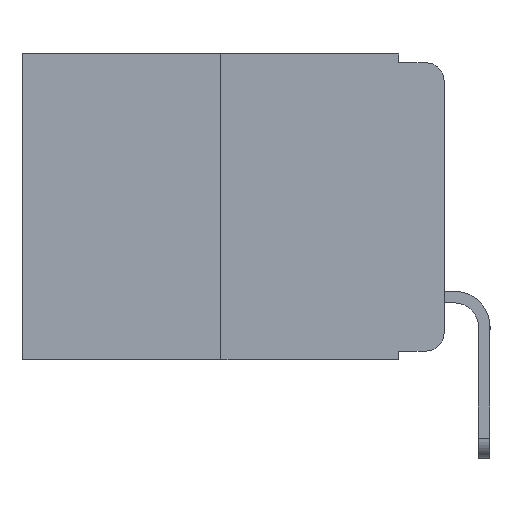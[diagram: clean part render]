
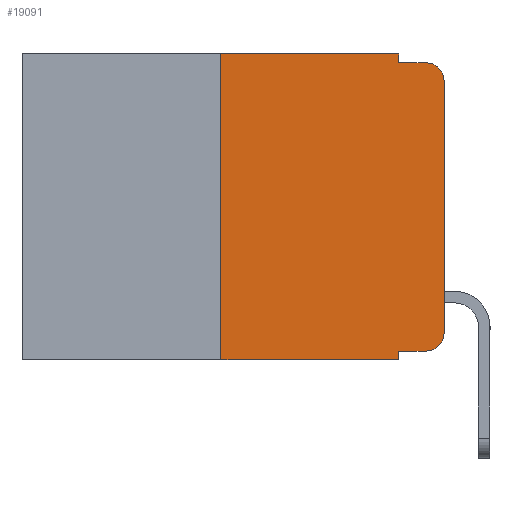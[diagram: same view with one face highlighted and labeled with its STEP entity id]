
A CAD part, left-side view. The second image highlights one B-rep face of the part: STEP entity #19091.
In plain terms, the highlighted planar face has unit normal (-1, 0, 0).
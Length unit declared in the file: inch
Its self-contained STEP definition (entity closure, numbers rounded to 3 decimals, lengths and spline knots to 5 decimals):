
#580 = LINE ( 'NONE', #835, #15946 ) ;
#835 = CARTESIAN_POINT ( 'NONE',  ( 0., 0.051, -0.01 ) ) ;
#1684 = VERTEX_POINT ( 'NONE', #20459 ) ;
#1889 = PLANE ( 'NONE',  #7330 ) ;
#2268 = EDGE_CURVE ( 'NONE', #1684, #6836, #22344, .T. ) ;
#2276 = DIRECTION ( 'NONE',  ( -1., 0., 0. ) ) ;
#2827 = VERTEX_POINT ( 'NONE', #14921 ) ;
#3112 = CARTESIAN_POINT ( 'NONE',  ( 0., 0., 0. ) ) ;
#3487 = CARTESIAN_POINT ( 'NONE',  ( 0., 0.25, -0.343 ) ) ;
#4690 = VECTOR ( 'NONE', #24886, 39.37008 ) ;
#4863 = CARTESIAN_POINT ( 'NONE',  ( 0., 0.02, -0.01 ) ) ;
#5251 = VECTOR ( 'NONE', #22073, 39.37008 ) ;
#5925 = LINE ( 'NONE', #6495, #5251 ) ;
#6188 = VECTOR ( 'NONE', #21374, 39.37008 ) ;
#6495 = CARTESIAN_POINT ( 'NONE',  ( 0., 0.473, -0.343 ) ) ;
#6691 = AXIS2_PLACEMENT_3D ( 'NONE', #9468, #22991, #11340 ) ;
#6836 = VERTEX_POINT ( 'NONE', #24330 ) ;
#7007 = VECTOR ( 'NONE', #13917, 39.37008 ) ;
#7330 = AXIS2_PLACEMENT_3D ( 'NONE', #16292, #10390, #23853 ) ;
#7694 = CARTESIAN_POINT ( 'NONE',  ( 0., 0.051, 0. ) ) ;
#8167 = EDGE_CURVE ( 'NONE', #10676, #2827, #22219, .T. ) ;
#8172 = EDGE_CURVE ( 'NONE', #2827, #24056, #17163, .T. ) ;
#8215 = EDGE_CURVE ( 'NONE', #19932, #24056, #580, .T. ) ;
#8297 = EDGE_CURVE ( 'NONE', #6836, #19932, #25761, .T. ) ;
#8474 = EDGE_CURVE ( 'NONE', #20167, #1684, #18103, .T. ) ;
#8585 = EDGE_CURVE ( 'NONE', #19271, #10582, #20757, .T. ) ;
#8639 = VERTEX_POINT ( 'NONE', #18443 ) ;
#8981 = CARTESIAN_POINT ( 'NONE',  ( 0., 0.051, -0.333 ) ) ;
#9074 = CIRCLE ( 'NONE', #20930, 0.02 ) ;
#9227 = EDGE_CURVE ( 'NONE', #19271, #8639, #18964, .T. ) ;
#9468 = CARTESIAN_POINT ( 'NONE',  ( 0., 0.02, -0.03 ) ) ;
#10390 = DIRECTION ( 'NONE',  ( 1., 0., 0. ) ) ;
#10391 = CARTESIAN_POINT ( 'NONE',  ( 0., 0.473, 0. ) ) ;
#10582 = VERTEX_POINT ( 'NONE', #19025 ) ;
#10676 = VERTEX_POINT ( 'NONE', #11258 ) ;
#11056 = ORIENTED_EDGE ( 'NONE', *, *, #8167, .T. ) ;
#11122 = ORIENTED_EDGE ( 'NONE', *, *, #8172, .T. ) ;
#11147 = ORIENTED_EDGE ( 'NONE', *, *, #8215, .F. ) ;
#11258 = CARTESIAN_POINT ( 'NONE',  ( 0., 0., -0.313 ) ) ;
#11340 = DIRECTION ( 'NONE',  ( 0., 0., -1. ) ) ;
#11666 = ORIENTED_EDGE ( 'NONE', *, *, #8297, .F. ) ;
#11766 = DIRECTION ( 'NONE',  ( 0., -1., 0. ) ) ;
#11786 = ORIENTED_EDGE ( 'NONE', *, *, #2268, .F. ) ;
#11795 = EDGE_CURVE ( 'NONE', #8639, #10676, #9074, .T. ) ;
#11841 = VECTOR ( 'NONE', #17309, 39.37008 ) ;
#12549 = ORIENTED_EDGE ( 'NONE', *, *, #8474, .F. ) ;
#13156 = ORIENTED_EDGE ( 'NONE', *, *, #20449, .T. ) ;
#13261 = ORIENTED_EDGE ( 'NONE', *, *, #8585, .F. ) ;
#13708 = VECTOR ( 'NONE', #11766, 39.37008 ) ;
#13917 = DIRECTION ( 'NONE',  ( 0., 0., 1. ) ) ;
#14631 = CARTESIAN_POINT ( 'NONE',  ( 0., 0.02, -0.313 ) ) ;
#14921 = CARTESIAN_POINT ( 'NONE',  ( 0., 0., -0.03 ) ) ;
#15043 = ORIENTED_EDGE ( 'NONE', *, *, #9227, .T. ) ;
#15085 = ORIENTED_EDGE ( 'NONE', *, *, #11795, .T. ) ;
#15946 = VECTOR ( 'NONE', #17407, 39.37008 ) ;
#16292 = CARTESIAN_POINT ( 'NONE',  ( 0., 0.473, 0. ) ) ;
#16586 = DIRECTION ( 'NONE',  ( 0., 0., -1. ) ) ;
#16919 = CARTESIAN_POINT ( 'NONE',  ( 0., 0.051, -0.01 ) ) ;
#17163 = CIRCLE ( 'NONE', #6691, 0.02 ) ;
#17309 = DIRECTION ( 'NONE',  ( 0., 0., 1. ) ) ;
#17407 = DIRECTION ( 'NONE',  ( 0., -1., 0. ) ) ;
#17725 = CARTESIAN_POINT ( 'NONE',  ( 0., 0.051, -0.333 ) ) ;
#18103 = LINE ( 'NONE', #19764, #7007 ) ;
#18443 = CARTESIAN_POINT ( 'NONE',  ( 0., 0.02, -0.333 ) ) ;
#18964 = LINE ( 'NONE', #17725, #13708 ) ;
#19025 = CARTESIAN_POINT ( 'NONE',  ( 0., 0.051, -0.343 ) ) ;
#19091 = ADVANCED_FACE ( 'NONE', ( #20760 ), #1889, .F. ) ;
#19271 = VERTEX_POINT ( 'NONE', #8981 ) ;
#19764 = CARTESIAN_POINT ( 'NONE',  ( 0., 0.25, 0. ) ) ;
#19932 = VERTEX_POINT ( 'NONE', #16919 ) ;
#20167 = VERTEX_POINT ( 'NONE', #3487 ) ;
#20449 = EDGE_CURVE ( 'NONE', #20167, #10582, #5925, .T. ) ;
#20459 = CARTESIAN_POINT ( 'NONE',  ( 0., 0.25, 0. ) ) ;
#20757 = LINE ( 'NONE', #21960, #24950 ) ;
#20760 = FACE_OUTER_BOUND ( 'NONE', #23395, .T. ) ;
#20930 = AXIS2_PLACEMENT_3D ( 'NONE', #14631, #2276, #16586 ) ;
#21374 = DIRECTION ( 'NONE',  ( 0., -1., 0. ) ) ;
#21960 = CARTESIAN_POINT ( 'NONE',  ( 0., 0.051, 0. ) ) ;
#22073 = DIRECTION ( 'NONE',  ( 0., -1., 0. ) ) ;
#22219 = LINE ( 'NONE', #3112, #11841 ) ;
#22344 = LINE ( 'NONE', #10391, #6188 ) ;
#22991 = DIRECTION ( 'NONE',  ( -1., 0., 0. ) ) ;
#23395 = EDGE_LOOP ( 'NONE', ( #11056, #11122, #11147, #11666, #11786, #12549, #13156, #13261, #15043, #15085 ) ) ;
#23750 = DIRECTION ( 'NONE',  ( 0., 0., -1. ) ) ;
#23853 = DIRECTION ( 'NONE',  ( 0., 0., -1. ) ) ;
#24056 = VERTEX_POINT ( 'NONE', #4863 ) ;
#24330 = CARTESIAN_POINT ( 'NONE',  ( 0., 0.051, 0. ) ) ;
#24886 = DIRECTION ( 'NONE',  ( 0., 0., -1. ) ) ;
#24950 = VECTOR ( 'NONE', #23750, 39.37008 ) ;
#25761 = LINE ( 'NONE', #7694, #4690 ) ;
